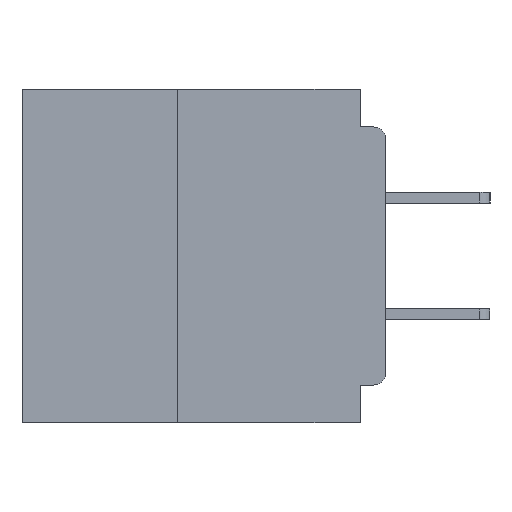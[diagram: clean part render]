
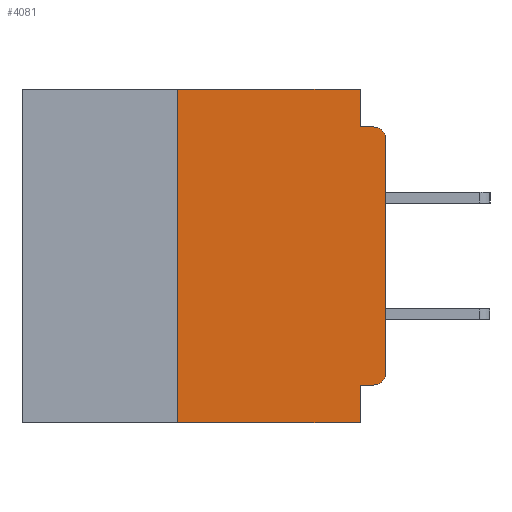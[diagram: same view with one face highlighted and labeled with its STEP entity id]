
A CAD part, left-side view. The second image highlights one B-rep face of the part: STEP entity #4081.
In plain terms, the highlighted planar face has unit normal (-1, 0, 0).
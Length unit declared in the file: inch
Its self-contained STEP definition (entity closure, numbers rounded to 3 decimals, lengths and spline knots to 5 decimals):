
#477 = CARTESIAN_POINT ( 'NONE',  ( 0., 0.015, -0.045 ) ) ;
#663 = EDGE_CURVE ( 'NONE', #26631, #26394, #32722, .T. ) ;
#2483 = DIRECTION ( 'NONE',  ( 0., 0., -1. ) ) ;
#2696 = CIRCLE ( 'NONE', #7538, 0.015 ) ;
#2856 = FACE_OUTER_BOUND ( 'NONE', #17339, .T. ) ;
#3980 = CARTESIAN_POINT ( 'NONE',  ( 0., 0.015, -0.34 ) ) ;
#4021 = VECTOR ( 'NONE', #29270, 39.37008 ) ;
#4081 = ADVANCED_FACE ( 'NONE', ( #2856 ), #36552, .F. ) ;
#4093 = VERTEX_POINT ( 'NONE', #35537 ) ;
#4240 = VECTOR ( 'NONE', #34582, 39.37008 ) ;
#4966 = DIRECTION ( 'NONE',  ( 0., 0., 1. ) ) ;
#5354 = LINE ( 'NONE', #34537, #22186 ) ;
#5944 = EDGE_CURVE ( 'NONE', #17854, #29146, #35442, .T. ) ;
#6143 = VERTEX_POINT ( 'NONE', #31229 ) ;
#6146 = ORIENTED_EDGE ( 'NONE', *, *, #5944, .F. ) ;
#6366 = EDGE_CURVE ( 'NONE', #29146, #32790, #20845, .T. ) ;
#6458 = ORIENTED_EDGE ( 'NONE', *, *, #14119, .T. ) ;
#7040 = DIRECTION ( 'NONE',  ( 0., 0., -1. ) ) ;
#7538 = AXIS2_PLACEMENT_3D ( 'NONE', #13958, #34421, #16934 ) ;
#7912 = CARTESIAN_POINT ( 'NONE',  ( 0., 0., -0.045 ) ) ;
#9828 = ORIENTED_EDGE ( 'NONE', *, *, #13603, .T. ) ;
#10162 = CARTESIAN_POINT ( 'NONE',  ( 0., 0., -0.355 ) ) ;
#10462 = VERTEX_POINT ( 'NONE', #28372 ) ;
#10602 = CARTESIAN_POINT ( 'NONE',  ( 0., 0.031, -0.045 ) ) ;
#10898 = VECTOR ( 'NONE', #16156, 39.37008 ) ;
#11496 = CARTESIAN_POINT ( 'NONE',  ( 0., 0.031, 0. ) ) ;
#12562 = AXIS2_PLACEMENT_3D ( 'NONE', #3980, #24837, #7040 ) ;
#13603 = EDGE_CURVE ( 'NONE', #18064, #4093, #19994, .T. ) ;
#13958 = CARTESIAN_POINT ( 'NONE',  ( 0., 0.015, -0.06 ) ) ;
#14119 = EDGE_CURVE ( 'NONE', #17704, #26394, #2696, .T. ) ;
#14508 = CARTESIAN_POINT ( 'NONE',  ( 0., 0.437, 0. ) ) ;
#15269 = DIRECTION ( 'NONE',  ( 0., -1., 0. ) ) ;
#16156 = DIRECTION ( 'NONE',  ( 0., 1., 0. ) ) ;
#16176 = EDGE_CURVE ( 'NONE', #4093, #17704, #5354, .T. ) ;
#16934 = DIRECTION ( 'NONE',  ( 0., 0., -1. ) ) ;
#17069 = CARTESIAN_POINT ( 'NONE',  ( 0., 0., -0.06 ) ) ;
#17339 = EDGE_LOOP ( 'NONE', ( #22129, #6458, #23330, #18002, #20227, #6146, #30659, #22370, #21858, #9828 ) ) ;
#17704 = VERTEX_POINT ( 'NONE', #17069 ) ;
#17832 = LINE ( 'NONE', #10162, #10898 ) ;
#17854 = VERTEX_POINT ( 'NONE', #20677 ) ;
#18002 = ORIENTED_EDGE ( 'NONE', *, *, #31709, .F. ) ;
#18064 = VERTEX_POINT ( 'NONE', #36287 ) ;
#19258 = VECTOR ( 'NONE', #21130, 39.37008 ) ;
#19994 = CIRCLE ( 'NONE', #12562, 0.015 ) ;
#20199 = LINE ( 'NONE', #32598, #19258 ) ;
#20227 = ORIENTED_EDGE ( 'NONE', *, *, #6366, .F. ) ;
#20547 = EDGE_CURVE ( 'NONE', #17854, #6143, #20199, .T. ) ;
#20677 = CARTESIAN_POINT ( 'NONE',  ( 0., 0.25, -0.4 ) ) ;
#20845 = LINE ( 'NONE', #14508, #27684 ) ;
#20983 = EDGE_CURVE ( 'NONE', #10462, #6143, #33835, .T. ) ;
#21130 = DIRECTION ( 'NONE',  ( 0., -1., 0. ) ) ;
#21858 = ORIENTED_EDGE ( 'NONE', *, *, #27155, .F. ) ;
#22129 = ORIENTED_EDGE ( 'NONE', *, *, #16176, .T. ) ;
#22186 = VECTOR ( 'NONE', #4966, 39.37008 ) ;
#22370 = ORIENTED_EDGE ( 'NONE', *, *, #20983, .F. ) ;
#23330 = ORIENTED_EDGE ( 'NONE', *, *, #663, .F. ) ;
#24093 = VECTOR ( 'NONE', #37793, 39.37008 ) ;
#24837 = DIRECTION ( 'NONE',  ( -1., 0., 0. ) ) ;
#25293 = CARTESIAN_POINT ( 'NONE',  ( 0., 0.25, 0. ) ) ;
#25599 = CARTESIAN_POINT ( 'NONE',  ( 0., 0.031, 0. ) ) ;
#26394 = VERTEX_POINT ( 'NONE', #477 ) ;
#26631 = VERTEX_POINT ( 'NONE', #10602 ) ;
#27155 = EDGE_CURVE ( 'NONE', #18064, #10462, #17832, .T. ) ;
#27678 = CARTESIAN_POINT ( 'NONE',  ( 0., 0.25, -0.4 ) ) ;
#27684 = VECTOR ( 'NONE', #15269, 39.37008 ) ;
#28372 = CARTESIAN_POINT ( 'NONE',  ( 0., 0.031, -0.355 ) ) ;
#29146 = VERTEX_POINT ( 'NONE', #25293 ) ;
#29270 = DIRECTION ( 'NONE',  ( 0., 0., 1. ) ) ;
#29316 = AXIS2_PLACEMENT_3D ( 'NONE', #38112, #36440, #36309 ) ;
#30213 = VECTOR ( 'NONE', #2483, 39.37008 ) ;
#30659 = ORIENTED_EDGE ( 'NONE', *, *, #20547, .T. ) ;
#31229 = CARTESIAN_POINT ( 'NONE',  ( 0., 0.031, -0.4 ) ) ;
#31709 = EDGE_CURVE ( 'NONE', #32790, #26631, #37903, .T. ) ;
#32598 = CARTESIAN_POINT ( 'NONE',  ( 0., 0.437, -0.4 ) ) ;
#32722 = LINE ( 'NONE', #7912, #24093 ) ;
#32790 = VERTEX_POINT ( 'NONE', #25599 ) ;
#33835 = LINE ( 'NONE', #34708, #4240 ) ;
#34421 = DIRECTION ( 'NONE',  ( -1., 0., 0. ) ) ;
#34537 = CARTESIAN_POINT ( 'NONE',  ( 0., 0., 0. ) ) ;
#34582 = DIRECTION ( 'NONE',  ( 0., 0., -1. ) ) ;
#34708 = CARTESIAN_POINT ( 'NONE',  ( 0., 0.031, -0.4 ) ) ;
#35442 = LINE ( 'NONE', #27678, #4021 ) ;
#35537 = CARTESIAN_POINT ( 'NONE',  ( 0., 0., -0.34 ) ) ;
#36287 = CARTESIAN_POINT ( 'NONE',  ( 0., 0.015, -0.355 ) ) ;
#36309 = DIRECTION ( 'NONE',  ( 0., 0., -1. ) ) ;
#36440 = DIRECTION ( 'NONE',  ( 1., 0., 0. ) ) ;
#36552 = PLANE ( 'NONE',  #29316 ) ;
#37793 = DIRECTION ( 'NONE',  ( 0., -1., 0. ) ) ;
#37903 = LINE ( 'NONE', #11496, #30213 ) ;
#38112 = CARTESIAN_POINT ( 'NONE',  ( 0., 0.437, 0. ) ) ;
